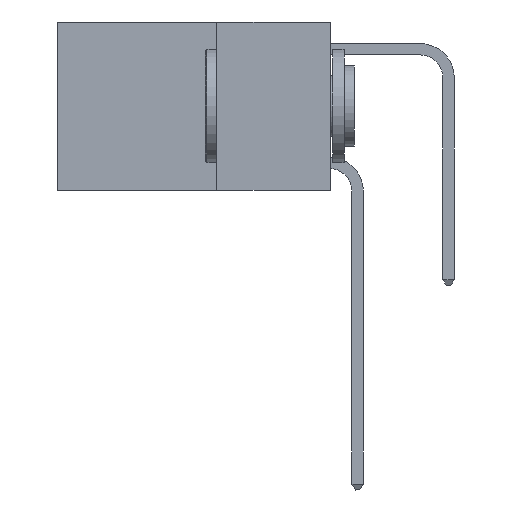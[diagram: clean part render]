
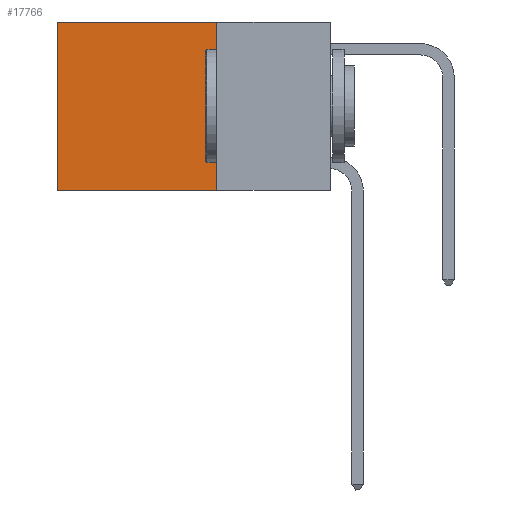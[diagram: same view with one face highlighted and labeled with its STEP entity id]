
A CAD part, left-side view. The second image highlights one B-rep face of the part: STEP entity #17766.
In plain terms, the highlighted planar face has unit normal (-1, 0, 0).
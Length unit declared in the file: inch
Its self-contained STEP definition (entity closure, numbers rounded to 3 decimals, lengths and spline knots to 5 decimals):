
#1250 = ORIENTED_EDGE ( 'NONE', *, *, #2700, .F. ) ;
#1539 = ORIENTED_EDGE ( 'NONE', *, *, #10616, .F. ) ;
#1682 = ORIENTED_EDGE ( 'NONE', *, *, #16750, .T. ) ;
#2498 = DIRECTION ( 'NONE',  ( 1., 0., 0. ) ) ;
#2700 = EDGE_CURVE ( 'NONE', #30411, #30520, #18693, .T. ) ;
#5137 = DIRECTION ( 'NONE',  ( 0., 0., -1. ) ) ;
#7532 = FACE_OUTER_BOUND ( 'NONE', #12022, .T. ) ;
#7896 = DIRECTION ( 'NONE',  ( 0., 1., 0. ) ) ;
#10295 = CARTESIAN_POINT ( 'NONE',  ( 0.2625, 0.25, 0. ) ) ;
#10616 = EDGE_CURVE ( 'NONE', #18986, #30411, #32230, .T. ) ;
#11797 = AXIS2_PLACEMENT_3D ( 'NONE', #10295, #2498, #20718 ) ;
#12022 = EDGE_LOOP ( 'NONE', ( #1682, #1250, #1539, #25840 ) ) ;
#14628 = LINE ( 'NONE', #23561, #21554 ) ;
#15377 = CARTESIAN_POINT ( 'NONE',  ( 0.2625, 0.6, 0. ) ) ;
#16101 = VECTOR ( 'NONE', #5137, 39.37008 ) ;
#16357 = CARTESIAN_POINT ( 'NONE',  ( 0.2625, 0.6, 0. ) ) ;
#16750 = EDGE_CURVE ( 'NONE', #33172, #30520, #23032, .T. ) ;
#17675 = CARTESIAN_POINT ( 'NONE',  ( 0.2625, 0.25, 0. ) ) ;
#17766 = ADVANCED_FACE ( 'NONE', ( #7532 ), #18099, .F. ) ;
#17874 = VECTOR ( 'NONE', #26172, 39.37008 ) ;
#18099 = PLANE ( 'NONE',  #11797 ) ;
#18693 = LINE ( 'NONE', #23546, #17874 ) ;
#18986 = VERTEX_POINT ( 'NONE', #17675 ) ;
#19356 = CARTESIAN_POINT ( 'NONE',  ( 0.2625, 0.25, -0.37 ) ) ;
#20718 = DIRECTION ( 'NONE',  ( 0., 0., -1. ) ) ;
#21554 = VECTOR ( 'NONE', #7896, 39.37008 ) ;
#23032 = LINE ( 'NONE', #15377, #16101 ) ;
#23546 = CARTESIAN_POINT ( 'NONE',  ( 0.2625, 0.25, -0.37 ) ) ;
#23561 = CARTESIAN_POINT ( 'NONE',  ( 0.2625, 0.25, 0. ) ) ;
#23816 = CARTESIAN_POINT ( 'NONE',  ( 0.2625, 0.25, 0. ) ) ;
#25840 = ORIENTED_EDGE ( 'NONE', *, *, #28332, .T. ) ;
#26172 = DIRECTION ( 'NONE',  ( 0., 1., 0. ) ) ;
#26440 = DIRECTION ( 'NONE',  ( 0., 0., -1. ) ) ;
#28142 = CARTESIAN_POINT ( 'NONE',  ( 0.2625, 0.6, -0.37 ) ) ;
#28332 = EDGE_CURVE ( 'NONE', #18986, #33172, #14628, .T. ) ;
#30411 = VERTEX_POINT ( 'NONE', #19356 ) ;
#30520 = VERTEX_POINT ( 'NONE', #28142 ) ;
#31446 = VECTOR ( 'NONE', #26440, 39.37008 ) ;
#32230 = LINE ( 'NONE', #23816, #31446 ) ;
#33172 = VERTEX_POINT ( 'NONE', #16357 ) ;
